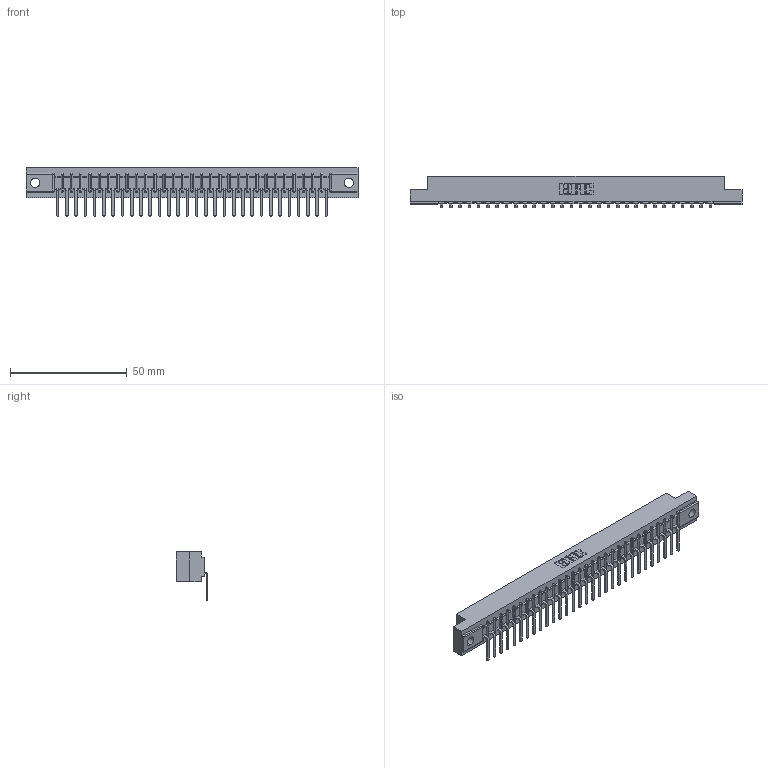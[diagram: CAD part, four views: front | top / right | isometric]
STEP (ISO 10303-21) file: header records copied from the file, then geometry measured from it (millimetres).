
FILE_DESCRIPTION (( 'STEP AP203' ), '1' );
FILE_NAME ('307-030-557-104.STEP', '2018-08-04T19:15:47', ( '' ), ( '' ), 'SwSTEP 2.0', 'SolidWorks 2016', '' );
FILE_SCHEMA (( 'CONFIG_CONTROL_DESIGN' ));
Length unit declared in the file: inch
Products named in the file (3): 307-290-002_557; 307-030-557-104; 307 Part_.156 Dia Mounting Holes
Assembly tree (31 placements, depth 2):
  307-030-557-104
    307 Part_.156 Dia Mounting Holes
    307-290-002_557  x30
Bounding box: 141.88 x 13.32 x 20.66 mm (x, y, z)
Volume: 15069 mm3; surface area: 19046.4 mm2
Topology: 31 solids, 31 shells, 2503 faces, 7679 edges, 5034 vertices
Faces by surface type: plane 1494, cylinder 947, sphere 62
Entity records: 28470 total; most frequent: CARTESIAN_POINT 4806, ORIENTED_EDGE 4794, DIRECTION 4667, EDGE_CURVE 2397, LINE 1837, VECTOR 1837, VERTEX_POINT 1554, AXIS2_PLACEMENT_3D 1415
